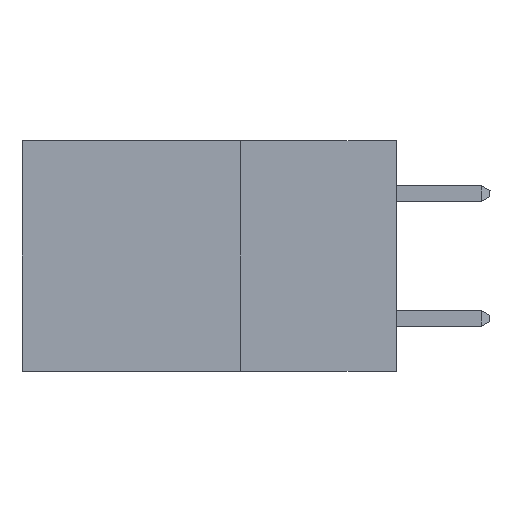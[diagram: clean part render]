
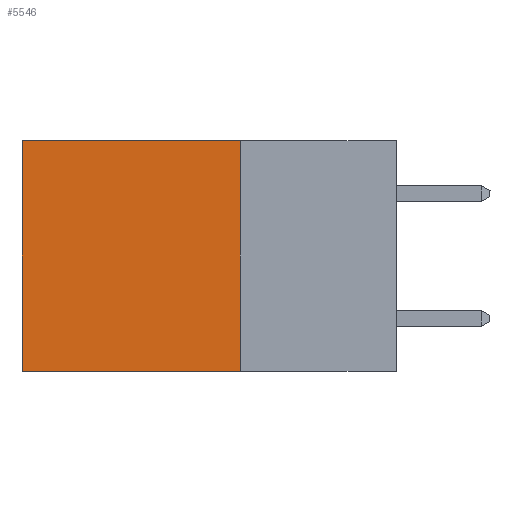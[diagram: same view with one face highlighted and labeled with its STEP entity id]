
A CAD part, left-side view. The second image highlights one B-rep face of the part: STEP entity #5546.
In plain terms, the highlighted planar face has unit normal (-1, 0, 0).
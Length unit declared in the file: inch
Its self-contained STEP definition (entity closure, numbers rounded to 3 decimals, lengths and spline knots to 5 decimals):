
#300 = VECTOR ( 'NONE', #7753, 39.37008 ) ;
#431 = CARTESIAN_POINT ( 'NONE',  ( 0.298, 0.25, -0.37 ) ) ;
#665 = LINE ( 'NONE', #7750, #300 ) ;
#1019 = EDGE_CURVE ( 'NONE', #2987, #5968, #7232, .T. ) ;
#1295 = LINE ( 'NONE', #4677, #5088 ) ;
#1326 = VECTOR ( 'NONE', #6760, 39.37008 ) ;
#1657 = EDGE_CURVE ( 'NONE', #2987, #4833, #1295, .T. ) ;
#1673 = LINE ( 'NONE', #2973, #7217 ) ;
#2155 = CARTESIAN_POINT ( 'NONE',  ( 0.298, 0.6, 0. ) ) ;
#2550 = EDGE_LOOP ( 'NONE', ( #12508, #7349, #11596, #4815 ) ) ;
#2973 = CARTESIAN_POINT ( 'NONE',  ( 0.298, 0.6, 0. ) ) ;
#2987 = VERTEX_POINT ( 'NONE', #8842 ) ;
#3025 = DIRECTION ( 'NONE',  ( 0., 0., -1. ) ) ;
#3568 = EDGE_CURVE ( 'NONE', #5968, #4888, #665, .T. ) ;
#3771 = FACE_OUTER_BOUND ( 'NONE', #2550, .T. ) ;
#4677 = CARTESIAN_POINT ( 'NONE',  ( 0.298, 0.25, 0. ) ) ;
#4815 = ORIENTED_EDGE ( 'NONE', *, *, #1657, .T. ) ;
#4833 = VERTEX_POINT ( 'NONE', #2155 ) ;
#4888 = VERTEX_POINT ( 'NONE', #11304 ) ;
#5088 = VECTOR ( 'NONE', #9893, 39.37008 ) ;
#5221 = CARTESIAN_POINT ( 'NONE',  ( 0.298, 0.25, 0. ) ) ;
#5228 = DIRECTION ( 'NONE',  ( 0., 0., -1. ) ) ;
#5546 = ADVANCED_FACE ( 'NONE', ( #3771 ), #7989, .F. ) ;
#5968 = VERTEX_POINT ( 'NONE', #431 ) ;
#6723 = EDGE_CURVE ( 'NONE', #4833, #4888, #1673, .T. ) ;
#6760 = DIRECTION ( 'NONE',  ( 0., 0., -1. ) ) ;
#7217 = VECTOR ( 'NONE', #3025, 39.37008 ) ;
#7232 = LINE ( 'NONE', #5221, #1326 ) ;
#7349 = ORIENTED_EDGE ( 'NONE', *, *, #3568, .F. ) ;
#7589 = DIRECTION ( 'NONE',  ( 1., 0., 0. ) ) ;
#7750 = CARTESIAN_POINT ( 'NONE',  ( 0.298, 0.25, -0.37 ) ) ;
#7753 = DIRECTION ( 'NONE',  ( 0., 1., 0. ) ) ;
#7956 = AXIS2_PLACEMENT_3D ( 'NONE', #8054, #7589, #5228 ) ;
#7989 = PLANE ( 'NONE',  #7956 ) ;
#8054 = CARTESIAN_POINT ( 'NONE',  ( 0.298, 0.25, 0. ) ) ;
#8842 = CARTESIAN_POINT ( 'NONE',  ( 0.298, 0.25, 0. ) ) ;
#9893 = DIRECTION ( 'NONE',  ( 0., 1., 0. ) ) ;
#11304 = CARTESIAN_POINT ( 'NONE',  ( 0.298, 0.6, -0.37 ) ) ;
#11596 = ORIENTED_EDGE ( 'NONE', *, *, #1019, .F. ) ;
#12508 = ORIENTED_EDGE ( 'NONE', *, *, #6723, .T. ) ;
